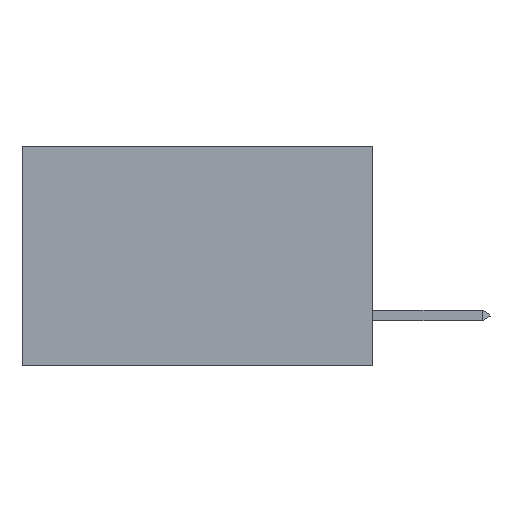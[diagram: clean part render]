
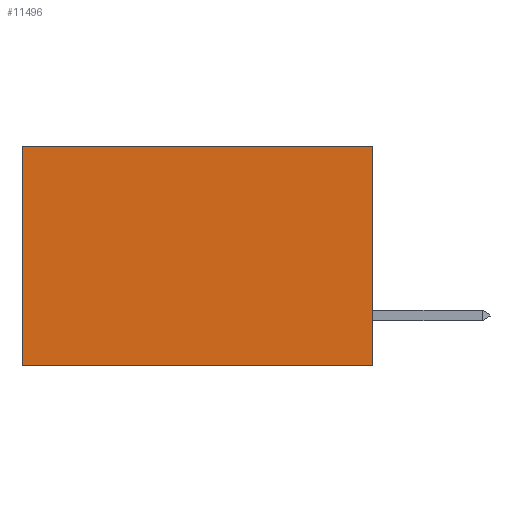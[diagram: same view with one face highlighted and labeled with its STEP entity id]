
A CAD part, left-side view. The second image highlights one B-rep face of the part: STEP entity #11496.
In plain terms, the highlighted planar face has unit normal (-1, 0, 0).
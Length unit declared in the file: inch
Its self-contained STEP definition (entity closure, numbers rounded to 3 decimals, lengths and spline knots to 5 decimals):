
#76 = AXIS2_PLACEMENT_3D ( 'NONE', #14964, #13218, #2590 ) ;
#1254 = LINE ( 'NONE', #20346, #4331 ) ;
#1723 = VERTEX_POINT ( 'NONE', #12296 ) ;
#2590 = DIRECTION ( 'NONE',  ( 0., 0., -1. ) ) ;
#3793 = EDGE_CURVE ( 'NONE', #22686, #13247, #7514, .T. ) ;
#3798 = ORIENTED_EDGE ( 'NONE', *, *, #6704, .F. ) ;
#4331 = VECTOR ( 'NONE', #20044, 39.37008 ) ;
#4746 = DIRECTION ( 'NONE',  ( 0., 0., -1. ) ) ;
#5466 = ORIENTED_EDGE ( 'NONE', *, *, #16273, .F. ) ;
#5954 = LINE ( 'NONE', #13620, #10140 ) ;
#6704 = EDGE_CURVE ( 'NONE', #22686, #11196, #1254, .T. ) ;
#7514 = LINE ( 'NONE', #10965, #16421 ) ;
#8448 = FACE_OUTER_BOUND ( 'NONE', #10245, .T. ) ;
#10140 = VECTOR ( 'NONE', #4746, 39.37008 ) ;
#10245 = EDGE_LOOP ( 'NONE', ( #18883, #5466, #3798, #20853 ) ) ;
#10877 = DIRECTION ( 'NONE',  ( 0., 1., 0. ) ) ;
#10965 = CARTESIAN_POINT ( 'NONE',  ( 0.277, 0., 0. ) ) ;
#11196 = VERTEX_POINT ( 'NONE', #15879 ) ;
#11496 = ADVANCED_FACE ( 'NONE', ( #8448 ), #20248, .F. ) ;
#12296 = CARTESIAN_POINT ( 'NONE',  ( 0.277, 0.59, -0.37 ) ) ;
#13218 = DIRECTION ( 'NONE',  ( 1., 0., 0. ) ) ;
#13247 = VERTEX_POINT ( 'NONE', #20896 ) ;
#13620 = CARTESIAN_POINT ( 'NONE',  ( 0.277, 0.59, -0.37 ) ) ;
#13774 = LINE ( 'NONE', #19373, #22583 ) ;
#14964 = CARTESIAN_POINT ( 'NONE',  ( 0.277, 0., -0.37 ) ) ;
#15221 = CARTESIAN_POINT ( 'NONE',  ( 0.277, 0., 0. ) ) ;
#15879 = CARTESIAN_POINT ( 'NONE',  ( 0.277, 0., -0.37 ) ) ;
#16273 = EDGE_CURVE ( 'NONE', #11196, #1723, #13774, .T. ) ;
#16421 = VECTOR ( 'NONE', #10877, 39.37008 ) ;
#18883 = ORIENTED_EDGE ( 'NONE', *, *, #21557, .T. ) ;
#19373 = CARTESIAN_POINT ( 'NONE',  ( 0.277, 0., -0.37 ) ) ;
#20044 = DIRECTION ( 'NONE',  ( 0., 0., -1. ) ) ;
#20248 = PLANE ( 'NONE',  #76 ) ;
#20346 = CARTESIAN_POINT ( 'NONE',  ( 0.277, 0., -0.37 ) ) ;
#20853 = ORIENTED_EDGE ( 'NONE', *, *, #3793, .T. ) ;
#20896 = CARTESIAN_POINT ( 'NONE',  ( 0.277, 0.59, 0. ) ) ;
#21118 = DIRECTION ( 'NONE',  ( 0., 1., 0. ) ) ;
#21557 = EDGE_CURVE ( 'NONE', #13247, #1723, #5954, .T. ) ;
#22583 = VECTOR ( 'NONE', #21118, 39.37008 ) ;
#22686 = VERTEX_POINT ( 'NONE', #15221 ) ;
